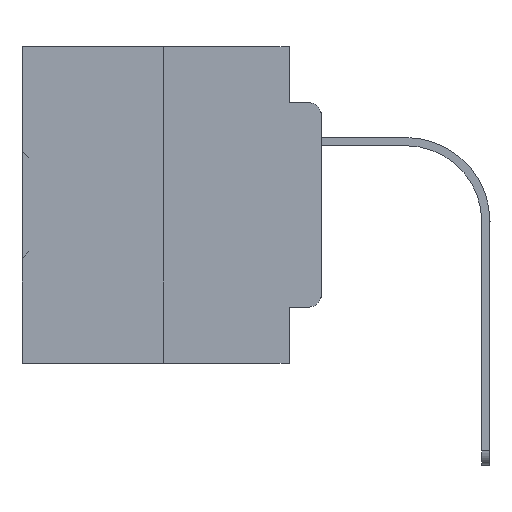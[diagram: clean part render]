
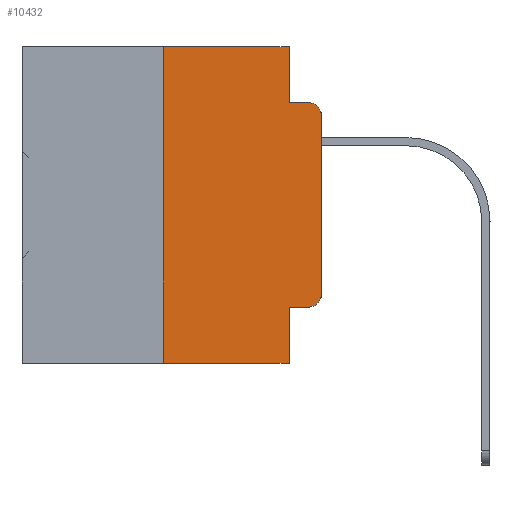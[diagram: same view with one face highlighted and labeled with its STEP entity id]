
A CAD part, left-side view. The second image highlights one B-rep face of the part: STEP entity #10432.
In plain terms, the highlighted planar face has unit normal (-1, 0, 0).
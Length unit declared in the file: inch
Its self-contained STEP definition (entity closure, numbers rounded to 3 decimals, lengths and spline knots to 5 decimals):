
#935 = LINE ( 'NONE', #35759, #25111 ) ;
#1234 = VERTEX_POINT ( 'NONE', #17129 ) ;
#1488 = VERTEX_POINT ( 'NONE', #36148 ) ;
#2365 = DIRECTION ( 'NONE',  ( 0., 0., -1. ) ) ;
#2456 = ORIENTED_EDGE ( 'NONE', *, *, #12148, .F. ) ;
#2699 = EDGE_CURVE ( 'NONE', #31754, #14873, #18273, .T. ) ;
#3398 = CARTESIAN_POINT ( 'NONE',  ( 0., 0.051, 0. ) ) ;
#3488 = VERTEX_POINT ( 'NONE', #9534 ) ;
#3501 = VECTOR ( 'NONE', #7953, 39.37008 ) ;
#4753 = EDGE_CURVE ( 'NONE', #7297, #3488, #10414, .T. ) ;
#5167 = ORIENTED_EDGE ( 'NONE', *, *, #20758, .F. ) ;
#5603 = CARTESIAN_POINT ( 'NONE',  ( 0., 0.25, -0.5 ) ) ;
#6172 = ORIENTED_EDGE ( 'NONE', *, *, #26371, .T. ) ;
#6277 = VERTEX_POINT ( 'NONE', #21324 ) ;
#7297 = VERTEX_POINT ( 'NONE', #37148 ) ;
#7641 = CARTESIAN_POINT ( 'NONE',  ( 0., 0., 0. ) ) ;
#7953 = DIRECTION ( 'NONE',  ( 0., -1., 0. ) ) ;
#9386 = LINE ( 'NONE', #3398, #30257 ) ;
#9422 = DIRECTION ( 'NONE',  ( 0., 0., -1. ) ) ;
#9534 = CARTESIAN_POINT ( 'NONE',  ( 0., 0.051, 0. ) ) ;
#10414 = LINE ( 'NONE', #21944, #25834 ) ;
#10432 = ADVANCED_FACE ( 'NONE', ( #14240 ), #16912, .F. ) ;
#10437 = ORIENTED_EDGE ( 'NONE', *, *, #15685, .F. ) ;
#12083 = DIRECTION ( 'NONE',  ( 0., 0., -1. ) ) ;
#12148 = EDGE_CURVE ( 'NONE', #6277, #1488, #33926, .T. ) ;
#12780 = VERTEX_POINT ( 'NONE', #21061 ) ;
#13069 = CARTESIAN_POINT ( 'NONE',  ( 0., 0.02, -0.3915 ) ) ;
#13487 = DIRECTION ( 'NONE',  ( 1., 0., 0. ) ) ;
#13610 = VERTEX_POINT ( 'NONE', #14966 ) ;
#13764 = DIRECTION ( 'NONE',  ( 0., 0., 1. ) ) ;
#14240 = FACE_OUTER_BOUND ( 'NONE', #14392, .T. ) ;
#14392 = EDGE_LOOP ( 'NONE', ( #21460, #26261, #2456, #25218, #30567, #10437, #23068, #5167, #34812, #6172 ) ) ;
#14873 = VERTEX_POINT ( 'NONE', #20022 ) ;
#14966 = CARTESIAN_POINT ( 'NONE',  ( 0., 0.02, -0.4115 ) ) ;
#15354 = DIRECTION ( 'NONE',  ( -1., 0., 0. ) ) ;
#15685 = EDGE_CURVE ( 'NONE', #31754, #7297, #22403, .T. ) ;
#15979 = DIRECTION ( 'NONE',  ( 0., -1., 0. ) ) ;
#16032 = AXIS2_PLACEMENT_3D ( 'NONE', #37130, #13487, #16355 ) ;
#16355 = DIRECTION ( 'NONE',  ( 0., 0., -1. ) ) ;
#16912 = PLANE ( 'NONE',  #16032 ) ;
#17129 = CARTESIAN_POINT ( 'NONE',  ( 0., 0., -0.1085 ) ) ;
#18085 = DIRECTION ( 'NONE',  ( 0., -1., 0. ) ) ;
#18273 = LINE ( 'NONE', #21158, #33865 ) ;
#18677 = EDGE_CURVE ( 'NONE', #34532, #1234, #36088, .T. ) ;
#18957 = DIRECTION ( 'NONE',  ( 0., -1., 0. ) ) ;
#20022 = CARTESIAN_POINT ( 'NONE',  ( 0., 0.051, -0.5 ) ) ;
#20263 = CARTESIAN_POINT ( 'NONE',  ( 0., 0.02, -0.1085 ) ) ;
#20758 = EDGE_CURVE ( 'NONE', #12780, #14873, #9386, .T. ) ;
#21061 = CARTESIAN_POINT ( 'NONE',  ( 0., 0.051, -0.4115 ) ) ;
#21158 = CARTESIAN_POINT ( 'NONE',  ( 0., 0.473, -0.5 ) ) ;
#21324 = CARTESIAN_POINT ( 'NONE',  ( 0., 0.051, -0.0885 ) ) ;
#21460 = ORIENTED_EDGE ( 'NONE', *, *, #18677, .T. ) ;
#21944 = CARTESIAN_POINT ( 'NONE',  ( 0., 0.473, 0. ) ) ;
#22403 = LINE ( 'NONE', #31229, #35141 ) ;
#23068 = ORIENTED_EDGE ( 'NONE', *, *, #2699, .T. ) ;
#25111 = VECTOR ( 'NONE', #9422, 39.37008 ) ;
#25218 = ORIENTED_EDGE ( 'NONE', *, *, #36421, .F. ) ;
#25834 = VECTOR ( 'NONE', #15979, 39.37008 ) ;
#26261 = ORIENTED_EDGE ( 'NONE', *, *, #28821, .T. ) ;
#26371 = EDGE_CURVE ( 'NONE', #13610, #34532, #36663, .T. ) ;
#27467 = DIRECTION ( 'NONE',  ( 0., 0., -1. ) ) ;
#27742 = VECTOR ( 'NONE', #18957, 39.37008 ) ;
#28821 = EDGE_CURVE ( 'NONE', #1234, #1488, #35529, .T. ) ;
#30257 = VECTOR ( 'NONE', #12083, 39.37008 ) ;
#30478 = CARTESIAN_POINT ( 'NONE',  ( 0., 0.051, -0.0885 ) ) ;
#30567 = ORIENTED_EDGE ( 'NONE', *, *, #4753, .F. ) ;
#31229 = CARTESIAN_POINT ( 'NONE',  ( 0., 0.25, 0. ) ) ;
#31754 = VERTEX_POINT ( 'NONE', #5603 ) ;
#31783 = DIRECTION ( 'NONE',  ( -1., 0., 0. ) ) ;
#32445 = AXIS2_PLACEMENT_3D ( 'NONE', #20263, #31783, #2365 ) ;
#32761 = CARTESIAN_POINT ( 'NONE',  ( 0., 0., -0.3915 ) ) ;
#33474 = VECTOR ( 'NONE', #36682, 39.37008 ) ;
#33865 = VECTOR ( 'NONE', #18085, 39.37008 ) ;
#33926 = LINE ( 'NONE', #30478, #27742 ) ;
#34270 = CARTESIAN_POINT ( 'NONE',  ( 0., 0.051, -0.4115 ) ) ;
#34532 = VERTEX_POINT ( 'NONE', #32761 ) ;
#34812 = ORIENTED_EDGE ( 'NONE', *, *, #34840, .T. ) ;
#34840 = EDGE_CURVE ( 'NONE', #12780, #13610, #36812, .T. ) ;
#35141 = VECTOR ( 'NONE', #13764, 39.37008 ) ;
#35529 = CIRCLE ( 'NONE', #32445, 0.02 ) ;
#35759 = CARTESIAN_POINT ( 'NONE',  ( 0., 0.051, 0. ) ) ;
#36088 = LINE ( 'NONE', #7641, #33474 ) ;
#36148 = CARTESIAN_POINT ( 'NONE',  ( 0., 0.02, -0.0885 ) ) ;
#36421 = EDGE_CURVE ( 'NONE', #3488, #6277, #935, .T. ) ;
#36663 = CIRCLE ( 'NONE', #37255, 0.02 ) ;
#36682 = DIRECTION ( 'NONE',  ( 0., 0., 1. ) ) ;
#36812 = LINE ( 'NONE', #34270, #3501 ) ;
#37130 = CARTESIAN_POINT ( 'NONE',  ( 0., 0.473, 0. ) ) ;
#37148 = CARTESIAN_POINT ( 'NONE',  ( 0., 0.25, 0. ) ) ;
#37255 = AXIS2_PLACEMENT_3D ( 'NONE', #13069, #15354, #27467 ) ;
